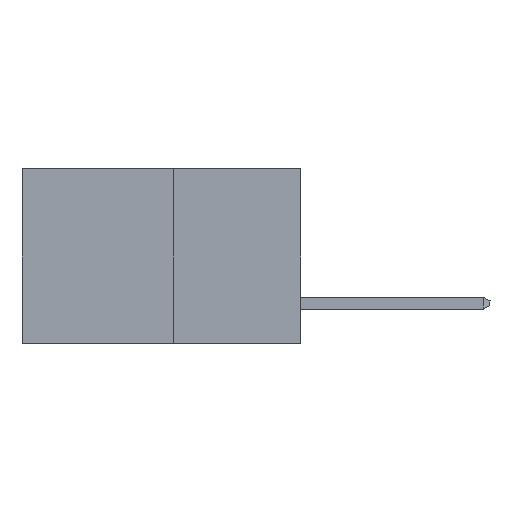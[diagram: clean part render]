
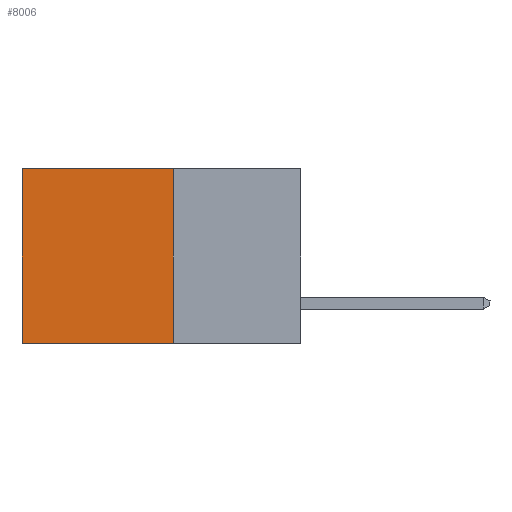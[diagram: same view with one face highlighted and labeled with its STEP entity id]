
A CAD part, left-side view. The second image highlights one B-rep face of the part: STEP entity #8006.
In plain terms, the highlighted planar face has unit normal (-1, 0, 0).
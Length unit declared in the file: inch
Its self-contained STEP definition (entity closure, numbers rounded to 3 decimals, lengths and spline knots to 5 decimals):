
#43 = VERTEX_POINT ( 'NONE', #5686 ) ;
#1420 = VECTOR ( 'NONE', #8197, 39.37008 ) ;
#1826 = DIRECTION ( 'NONE',  ( 0., 0., -1. ) ) ;
#2422 = LINE ( 'NONE', #8897, #4965 ) ;
#3478 = EDGE_CURVE ( 'NONE', #10432, #7141, #2422, .T. ) ;
#3691 = EDGE_CURVE ( 'NONE', #10432, #43, #9039, .T. ) ;
#3696 = DIRECTION ( 'NONE',  ( 0., 0., -1. ) ) ;
#3922 = CARTESIAN_POINT ( 'NONE',  ( 0.277, 0.27, -0.37 ) ) ;
#4233 = CARTESIAN_POINT ( 'NONE',  ( 0.277, 0.59, 0. ) ) ;
#4440 = FACE_OUTER_BOUND ( 'NONE', #6737, .T. ) ;
#4443 = EDGE_CURVE ( 'NONE', #7141, #5242, #10223, .T. ) ;
#4918 = CARTESIAN_POINT ( 'NONE',  ( 0.277, 0.59, -0.37 ) ) ;
#4965 = VECTOR ( 'NONE', #7285, 39.37008 ) ;
#5242 = VERTEX_POINT ( 'NONE', #4918 ) ;
#5648 = CARTESIAN_POINT ( 'NONE',  ( 0.277, 0.27, 0. ) ) ;
#5686 = CARTESIAN_POINT ( 'NONE',  ( 0.277, 0.27, -0.37 ) ) ;
#6737 = EDGE_LOOP ( 'NONE', ( #10819, #7136, #7116, #7021 ) ) ;
#6787 = VECTOR ( 'NONE', #1826, 39.37008 ) ;
#6877 = EDGE_CURVE ( 'NONE', #43, #5242, #10762, .T. ) ;
#7021 = ORIENTED_EDGE ( 'NONE', *, *, #3478, .T. ) ;
#7116 = ORIENTED_EDGE ( 'NONE', *, *, #3691, .F. ) ;
#7136 = ORIENTED_EDGE ( 'NONE', *, *, #6877, .F. ) ;
#7141 = VERTEX_POINT ( 'NONE', #4233 ) ;
#7285 = DIRECTION ( 'NONE',  ( 0., 1., 0. ) ) ;
#7297 = CARTESIAN_POINT ( 'NONE',  ( 0.277, 0.27, -0.37 ) ) ;
#7579 = DIRECTION ( 'NONE',  ( 0., 0., -1. ) ) ;
#7641 = AXIS2_PLACEMENT_3D ( 'NONE', #7297, #8974, #3696 ) ;
#7771 = CARTESIAN_POINT ( 'NONE',  ( 0.277, 0.59, -0.37 ) ) ;
#8006 = ADVANCED_FACE ( 'NONE', ( #4440 ), #8140, .F. ) ;
#8097 = VECTOR ( 'NONE', #7579, 39.37008 ) ;
#8140 = PLANE ( 'NONE',  #7641 ) ;
#8197 = DIRECTION ( 'NONE',  ( 0., 1., 0. ) ) ;
#8219 = CARTESIAN_POINT ( 'NONE',  ( 0.277, 0.27, -0.37 ) ) ;
#8897 = CARTESIAN_POINT ( 'NONE',  ( 0.277, 0.27, 0. ) ) ;
#8974 = DIRECTION ( 'NONE',  ( 1., 0., 0. ) ) ;
#9039 = LINE ( 'NONE', #3922, #6787 ) ;
#10223 = LINE ( 'NONE', #7771, #8097 ) ;
#10432 = VERTEX_POINT ( 'NONE', #5648 ) ;
#10762 = LINE ( 'NONE', #8219, #1420 ) ;
#10819 = ORIENTED_EDGE ( 'NONE', *, *, #4443, .T. ) ;
